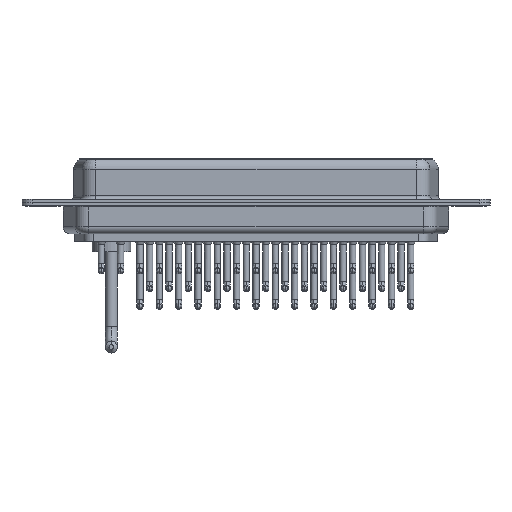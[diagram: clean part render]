
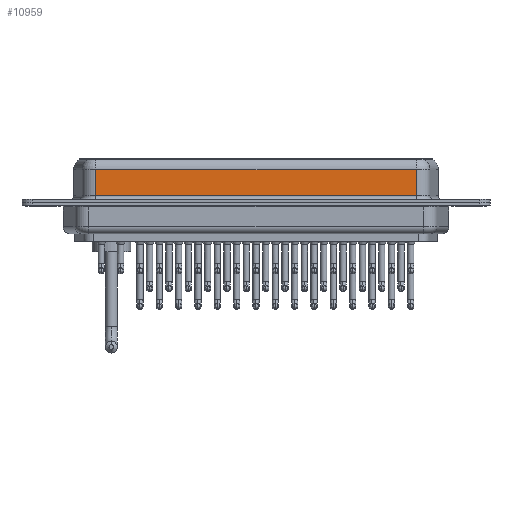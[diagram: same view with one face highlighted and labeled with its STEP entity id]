
A CAD part, front view. The second image highlights one B-rep face of the part: STEP entity #10959.
In plain terms, the highlighted planar face has unit normal (0, -1, 0).
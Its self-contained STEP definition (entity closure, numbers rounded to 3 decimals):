
#155 = LINE ( 'NONE', #27185, #17422 ) ;
#1391 = VECTOR ( 'NONE', #27378, 1000. ) ;
#3325 = CARTESIAN_POINT ( 'NONE',  ( 7.59, -5.375, 6.4 ) ) ;
#3762 = VECTOR ( 'NONE', #20310, 1000. ) ;
#5002 = EDGE_CURVE ( 'NONE', #9739, #6092, #25681, .T. ) ;
#6092 = VERTEX_POINT ( 'NONE', #23329 ) ;
#7042 = ORIENTED_EDGE ( 'NONE', *, *, #23677, .T. ) ;
#8553 = VERTEX_POINT ( 'NONE', #22689 ) ;
#9410 = EDGE_CURVE ( 'NONE', #9739, #18774, #155, .T. ) ;
#9449 = PLANE ( 'NONE',  #15955 ) ;
#9683 = LINE ( 'NONE', #14541, #1391 ) ;
#9739 = VERTEX_POINT ( 'NONE', #29392 ) ;
#10097 = DIRECTION ( 'NONE',  ( -1., 0., 0. ) ) ;
#10244 = CARTESIAN_POINT ( 'NONE',  ( 53.41, -5.375, 6.4 ) ) ;
#10959 = ADVANCED_FACE ( 'NONE', ( #14297 ), #9449, .F. ) ;
#12445 = CARTESIAN_POINT ( 'NONE',  ( 7.59, -5.375, 4.65 ) ) ;
#13711 = DIRECTION ( 'NONE',  ( 0., 0., -1. ) ) ;
#14010 = VECTOR ( 'NONE', #13711, 1000. ) ;
#14297 = FACE_OUTER_BOUND ( 'NONE', #22687, .T. ) ;
#14541 = CARTESIAN_POINT ( 'NONE',  ( 53.41, -5.375, 0.9 ) ) ;
#15955 = AXIS2_PLACEMENT_3D ( 'NONE', #16404, #24567, #26521 ) ;
#16404 = CARTESIAN_POINT ( 'NONE',  ( 53.41, -5.375, 6.4 ) ) ;
#17422 = VECTOR ( 'NONE', #10097, 1000. ) ;
#18774 = VERTEX_POINT ( 'NONE', #12445 ) ;
#20310 = DIRECTION ( 'NONE',  ( 0., 0., -1. ) ) ;
#22687 = EDGE_LOOP ( 'NONE', ( #24940, #29905, #7042, #31564 ) ) ;
#22689 = CARTESIAN_POINT ( 'NONE',  ( 7.59, -5.375, 0.9 ) ) ;
#23329 = CARTESIAN_POINT ( 'NONE',  ( 53.41, -5.375, 0.9 ) ) ;
#23677 = EDGE_CURVE ( 'NONE', #18774, #8553, #25606, .T. ) ;
#24567 = DIRECTION ( 'NONE',  ( 0., 1., 0. ) ) ;
#24940 = ORIENTED_EDGE ( 'NONE', *, *, #5002, .F. ) ;
#25606 = LINE ( 'NONE', #3325, #14010 ) ;
#25681 = LINE ( 'NONE', #10244, #3762 ) ;
#26521 = DIRECTION ( 'NONE',  ( 0., 0., 1. ) ) ;
#27185 = CARTESIAN_POINT ( 'NONE',  ( 53.41, -5.375, 4.65 ) ) ;
#27378 = DIRECTION ( 'NONE',  ( 1., 0., 0. ) ) ;
#29392 = CARTESIAN_POINT ( 'NONE',  ( 53.41, -5.375, 4.65 ) ) ;
#29905 = ORIENTED_EDGE ( 'NONE', *, *, #9410, .T. ) ;
#30063 = EDGE_CURVE ( 'NONE', #8553, #6092, #9683, .T. ) ;
#31564 = ORIENTED_EDGE ( 'NONE', *, *, #30063, .T. ) ;
